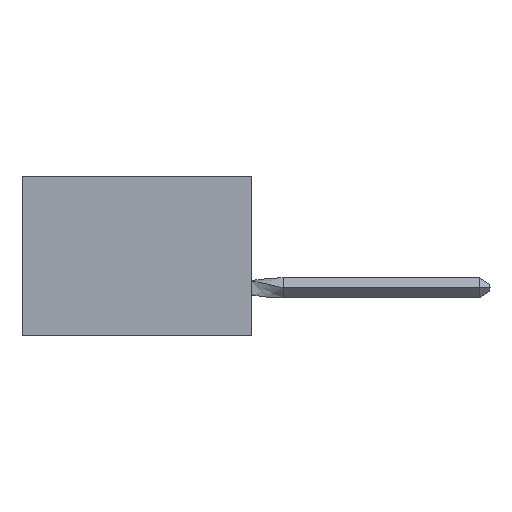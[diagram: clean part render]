
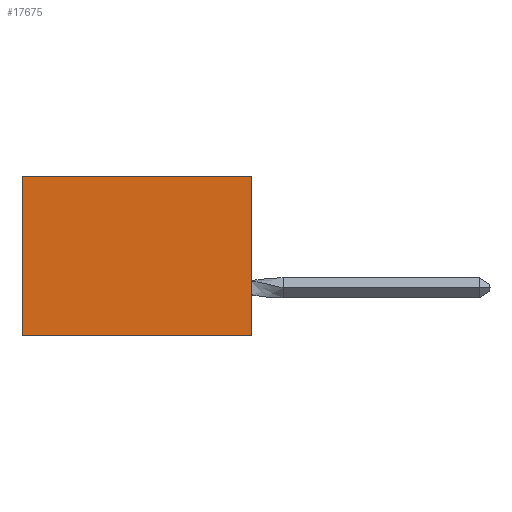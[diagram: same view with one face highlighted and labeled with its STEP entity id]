
A CAD part, left-side view. The second image highlights one B-rep face of the part: STEP entity #17675.
In plain terms, the highlighted planar face has unit normal (-1, 0, 0).
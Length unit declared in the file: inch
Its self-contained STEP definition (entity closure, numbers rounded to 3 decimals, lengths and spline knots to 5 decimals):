
#1015 = VERTEX_POINT ( 'NONE', #17044 ) ;
#1091 = EDGE_LOOP ( 'NONE', ( #10903, #12827, #1838, #7888 ) ) ;
#1652 = CARTESIAN_POINT ( 'NONE',  ( 0.305, 0., -0.5 ) ) ;
#1838 = ORIENTED_EDGE ( 'NONE', *, *, #20670, .F. ) ;
#2357 = DIRECTION ( 'NONE',  ( 0., 1., 0. ) ) ;
#2579 = FACE_OUTER_BOUND ( 'NONE', #1091, .T. ) ;
#4718 = EDGE_CURVE ( 'NONE', #9728, #1015, #11294, .T. ) ;
#5644 = LINE ( 'NONE', #8221, #5864 ) ;
#5864 = VECTOR ( 'NONE', #14836, 39.37008 ) ;
#5899 = CARTESIAN_POINT ( 'NONE',  ( 0.305, 0.72, -0.5 ) ) ;
#6567 = VECTOR ( 'NONE', #8813, 39.37008 ) ;
#6815 = DIRECTION ( 'NONE',  ( 1., 0., 0. ) ) ;
#6824 = LINE ( 'NONE', #1652, #18756 ) ;
#7043 = DIRECTION ( 'NONE',  ( 0., 0., -1. ) ) ;
#7281 = EDGE_CURVE ( 'NONE', #16946, #15157, #5644, .T. ) ;
#7888 = ORIENTED_EDGE ( 'NONE', *, *, #4718, .T. ) ;
#8221 = CARTESIAN_POINT ( 'NONE',  ( 0.305, 0., -0.5 ) ) ;
#8519 = VECTOR ( 'NONE', #2357, 39.37008 ) ;
#8554 = CARTESIAN_POINT ( 'NONE',  ( 0.305, 0., 0. ) ) ;
#8813 = DIRECTION ( 'NONE',  ( 0., 0., -1. ) ) ;
#9526 = CARTESIAN_POINT ( 'NONE',  ( 0.305, 0., -0.5 ) ) ;
#9728 = VERTEX_POINT ( 'NONE', #15804 ) ;
#10903 = ORIENTED_EDGE ( 'NONE', *, *, #11985, .T. ) ;
#11294 = LINE ( 'NONE', #8554, #8519 ) ;
#11712 = CARTESIAN_POINT ( 'NONE',  ( 0.305, 0., -0.5 ) ) ;
#11985 = EDGE_CURVE ( 'NONE', #1015, #15157, #16971, .T. ) ;
#11991 = PLANE ( 'NONE',  #18710 ) ;
#12827 = ORIENTED_EDGE ( 'NONE', *, *, #7281, .F. ) ;
#12855 = DIRECTION ( 'NONE',  ( 0., 0., -1. ) ) ;
#13762 = CARTESIAN_POINT ( 'NONE',  ( 0.305, 0.72, -0.5 ) ) ;
#14836 = DIRECTION ( 'NONE',  ( 0., 1., 0. ) ) ;
#15157 = VERTEX_POINT ( 'NONE', #5899 ) ;
#15804 = CARTESIAN_POINT ( 'NONE',  ( 0.305, 0., 0. ) ) ;
#16946 = VERTEX_POINT ( 'NONE', #9526 ) ;
#16971 = LINE ( 'NONE', #13762, #6567 ) ;
#17044 = CARTESIAN_POINT ( 'NONE',  ( 0.305, 0.72, 0. ) ) ;
#17675 = ADVANCED_FACE ( 'NONE', ( #2579 ), #11991, .F. ) ;
#18710 = AXIS2_PLACEMENT_3D ( 'NONE', #11712, #6815, #7043 ) ;
#18756 = VECTOR ( 'NONE', #12855, 39.37008 ) ;
#20670 = EDGE_CURVE ( 'NONE', #9728, #16946, #6824, .T. ) ;
